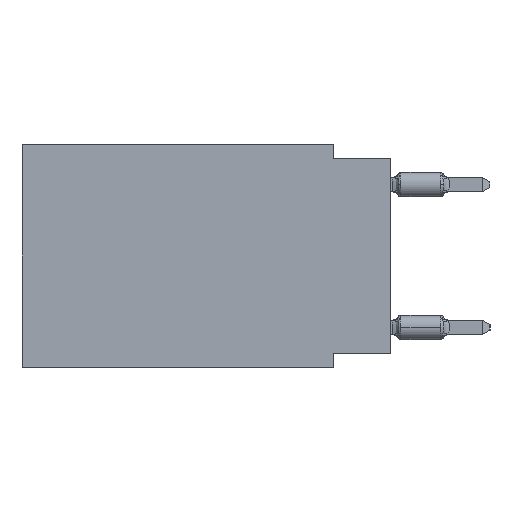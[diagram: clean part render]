
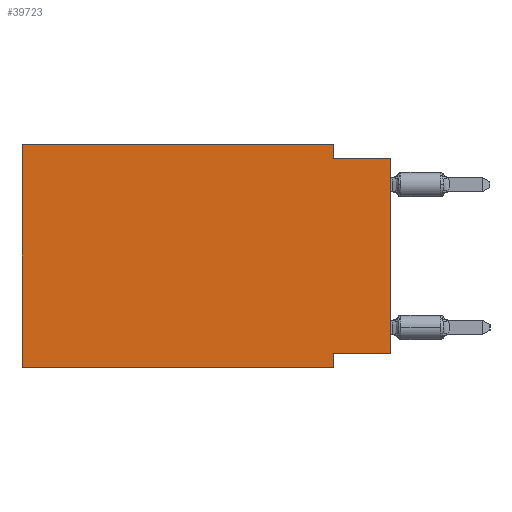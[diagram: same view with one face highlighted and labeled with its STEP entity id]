
A CAD part, left-side view. The second image highlights one B-rep face of the part: STEP entity #39723.
In plain terms, the highlighted planar face has unit normal (-1, 0, 0).
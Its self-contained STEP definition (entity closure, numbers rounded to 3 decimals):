
#455 = EDGE_CURVE ( 'NONE', #24078, #5617, #27369, .T. ) ;
#1613 = ORIENTED_EDGE ( 'NONE', *, *, #3512, .F. ) ;
#3512 = EDGE_CURVE ( 'NONE', #33217, #5617, #26774, .T. ) ;
#4298 = CARTESIAN_POINT ( 'NONE',  ( 0., 16.383, 0. ) ) ;
#4484 = EDGE_CURVE ( 'NONE', #8299, #25201, #41064, .T. ) ;
#4906 = ORIENTED_EDGE ( 'NONE', *, *, #19786, .F. ) ;
#4979 = EDGE_CURVE ( 'NONE', #27705, #33217, #9831, .T. ) ;
#5617 = VERTEX_POINT ( 'NONE', #51136 ) ;
#5683 = EDGE_CURVE ( 'NONE', #24078, #36543, #17543, .T. ) ;
#7329 = VECTOR ( 'NONE', #44809, 1000. ) ;
#8245 = DIRECTION ( 'NONE',  ( 0., 0., 1. ) ) ;
#8299 = VERTEX_POINT ( 'NONE', #32652 ) ;
#8556 = CARTESIAN_POINT ( 'NONE',  ( 0., 0., 0. ) ) ;
#8579 = VECTOR ( 'NONE', #19344, 1000. ) ;
#9831 = LINE ( 'NONE', #10138, #12506 ) ;
#10138 = CARTESIAN_POINT ( 'NONE',  ( 0., 2.54, 0. ) ) ;
#11157 = ORIENTED_EDGE ( 'NONE', *, *, #4979, .F. ) ;
#11460 = DIRECTION ( 'NONE',  ( 0., 0., -1. ) ) ;
#12344 = FACE_OUTER_BOUND ( 'NONE', #33018, .T. ) ;
#12506 = VECTOR ( 'NONE', #29273, 1000. ) ;
#12519 = DIRECTION ( 'NONE',  ( 0., -1., 0. ) ) ;
#14378 = CARTESIAN_POINT ( 'NONE',  ( 0., 0., -9.271 ) ) ;
#15034 = VECTOR ( 'NONE', #11460, 1000. ) ;
#16891 = CARTESIAN_POINT ( 'NONE',  ( 0., 2.54, -9.906 ) ) ;
#17226 = CARTESIAN_POINT ( 'NONE',  ( 0., 16.383, -9.906 ) ) ;
#17543 = LINE ( 'NONE', #14378, #8579 ) ;
#19344 = DIRECTION ( 'NONE',  ( 0., 1., 0. ) ) ;
#19564 = CARTESIAN_POINT ( 'NONE',  ( 0., 2.54, -0.635 ) ) ;
#19786 = EDGE_CURVE ( 'NONE', #53759, #27705, #50882, .T. ) ;
#22971 = ORIENTED_EDGE ( 'NONE', *, *, #32866, .F. ) ;
#23392 = VECTOR ( 'NONE', #30865, 1000. ) ;
#24078 = VERTEX_POINT ( 'NONE', #37791 ) ;
#25201 = VERTEX_POINT ( 'NONE', #16891 ) ;
#26448 = DIRECTION ( 'NONE',  ( 1., 0., 0. ) ) ;
#26754 = DIRECTION ( 'NONE',  ( 0., 0., -1. ) ) ;
#26774 = LINE ( 'NONE', #50029, #23392 ) ;
#27369 = LINE ( 'NONE', #8556, #28164 ) ;
#27705 = VERTEX_POINT ( 'NONE', #61041 ) ;
#28164 = VECTOR ( 'NONE', #8245, 1000. ) ;
#29273 = DIRECTION ( 'NONE',  ( 0., 0., -1. ) ) ;
#29615 = ORIENTED_EDGE ( 'NONE', *, *, #455, .T. ) ;
#30079 = LINE ( 'NONE', #54873, #7329 ) ;
#30507 = AXIS2_PLACEMENT_3D ( 'NONE', #50629, #26448, #26754 ) ;
#30865 = DIRECTION ( 'NONE',  ( 0., -1., 0. ) ) ;
#31517 = LINE ( 'NONE', #50679, #15034 ) ;
#31970 = ORIENTED_EDGE ( 'NONE', *, *, #5683, .F. ) ;
#32233 = CARTESIAN_POINT ( 'NONE',  ( 0., 2.54, -9.271 ) ) ;
#32652 = CARTESIAN_POINT ( 'NONE',  ( 0., 16.383, -9.906 ) ) ;
#32866 = EDGE_CURVE ( 'NONE', #36543, #25201, #31517, .T. ) ;
#33018 = EDGE_LOOP ( 'NONE', ( #29615, #1613, #11157, #4906, #46092, #39573, #22971, #31970 ) ) ;
#33217 = VERTEX_POINT ( 'NONE', #19564 ) ;
#36412 = EDGE_CURVE ( 'NONE', #8299, #53759, #30079, .T. ) ;
#36543 = VERTEX_POINT ( 'NONE', #32233 ) ;
#37791 = CARTESIAN_POINT ( 'NONE',  ( 0., 0., -9.271 ) ) ;
#39573 = ORIENTED_EDGE ( 'NONE', *, *, #4484, .T. ) ;
#39723 = ADVANCED_FACE ( 'NONE', ( #12344 ), #54711, .F. ) ;
#41064 = LINE ( 'NONE', #17226, #56568 ) ;
#44802 = VECTOR ( 'NONE', #55900, 1000. ) ;
#44809 = DIRECTION ( 'NONE',  ( 0., 0., 1. ) ) ;
#46092 = ORIENTED_EDGE ( 'NONE', *, *, #36412, .F. ) ;
#50029 = CARTESIAN_POINT ( 'NONE',  ( 0., 0., -0.635 ) ) ;
#50629 = CARTESIAN_POINT ( 'NONE',  ( 0., 16.383, 0. ) ) ;
#50679 = CARTESIAN_POINT ( 'NONE',  ( 0., 2.54, -9.906 ) ) ;
#50882 = LINE ( 'NONE', #51512, #44802 ) ;
#51136 = CARTESIAN_POINT ( 'NONE',  ( 0., 0., -0.635 ) ) ;
#51512 = CARTESIAN_POINT ( 'NONE',  ( 0., 16.383, 0. ) ) ;
#53759 = VERTEX_POINT ( 'NONE', #4298 ) ;
#54711 = PLANE ( 'NONE',  #30507 ) ;
#54873 = CARTESIAN_POINT ( 'NONE',  ( 0., 16.383, 0. ) ) ;
#55900 = DIRECTION ( 'NONE',  ( 0., -1., 0. ) ) ;
#56568 = VECTOR ( 'NONE', #12519, 1000. ) ;
#61041 = CARTESIAN_POINT ( 'NONE',  ( 0., 2.54, 0. ) ) ;
